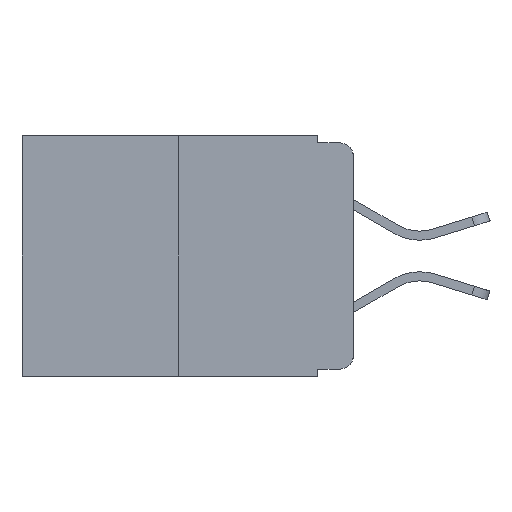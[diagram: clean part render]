
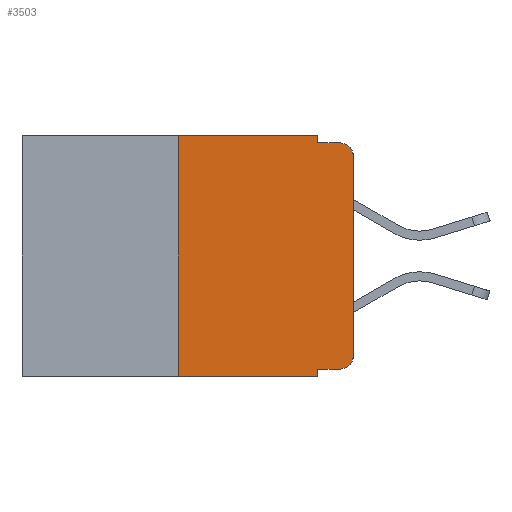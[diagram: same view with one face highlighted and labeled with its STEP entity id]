
A CAD part, left-side view. The second image highlights one B-rep face of the part: STEP entity #3503.
In plain terms, the highlighted planar face has unit normal (-1, 0, 0).
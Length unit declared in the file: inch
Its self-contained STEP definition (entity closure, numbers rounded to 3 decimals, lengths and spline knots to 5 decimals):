
#55 = LINE ( 'NONE', #13478, #4183 ) ;
#272 = DIRECTION ( 'NONE',  ( 0., 0., 1. ) ) ;
#337 = AXIS2_PLACEMENT_3D ( 'NONE', #536, #3952, #6984 ) ;
#490 = ORIENTED_EDGE ( 'NONE', *, *, #3819, .T. ) ;
#536 = CARTESIAN_POINT ( 'NONE',  ( 0., 0.02, -0.313 ) ) ;
#704 = DIRECTION ( 'NONE',  ( 1., 0., 0. ) ) ;
#1139 = AXIS2_PLACEMENT_3D ( 'NONE', #10734, #704, #8183 ) ;
#1156 = VERTEX_POINT ( 'NONE', #13085 ) ;
#1263 = CARTESIAN_POINT ( 'NONE',  ( 0., 0.051, -0.01 ) ) ;
#1621 = CARTESIAN_POINT ( 'NONE',  ( 0., 0., -0.03 ) ) ;
#1637 = CARTESIAN_POINT ( 'NONE',  ( 0., 0.25, -0.343 ) ) ;
#1801 = PLANE ( 'NONE',  #1139 ) ;
#2365 = DIRECTION ( 'NONE',  ( 0., -1., 0. ) ) ;
#2472 = DIRECTION ( 'NONE',  ( 0., -1., 0. ) ) ;
#2976 = VERTEX_POINT ( 'NONE', #6078 ) ;
#3007 = DIRECTION ( 'NONE',  ( 0., 0., -1. ) ) ;
#3343 = VERTEX_POINT ( 'NONE', #11411 ) ;
#3503 = ADVANCED_FACE ( 'NONE', ( #11851 ), #1801, .F. ) ;
#3701 = ORIENTED_EDGE ( 'NONE', *, *, #7362, .T. ) ;
#3819 = EDGE_CURVE ( 'NONE', #2976, #9929, #55, .T. ) ;
#3894 = CARTESIAN_POINT ( 'NONE',  ( 0., 0.02, -0.333 ) ) ;
#3932 = VERTEX_POINT ( 'NONE', #1637 ) ;
#3952 = DIRECTION ( 'NONE',  ( -1., 0., 0. ) ) ;
#4183 = VECTOR ( 'NONE', #272, 39.37008 ) ;
#4614 = AXIS2_PLACEMENT_3D ( 'NONE', #6065, #12837, #7255 ) ;
#4623 = LINE ( 'NONE', #1263, #12595 ) ;
#4680 = ORIENTED_EDGE ( 'NONE', *, *, #5674, .F. ) ;
#5674 = EDGE_CURVE ( 'NONE', #7776, #1156, #10786, .T. ) ;
#6061 = CARTESIAN_POINT ( 'NONE',  ( 0., 0.051, 0. ) ) ;
#6065 = CARTESIAN_POINT ( 'NONE',  ( 0., 0.02, -0.03 ) ) ;
#6078 = CARTESIAN_POINT ( 'NONE',  ( 0., 0., -0.313 ) ) ;
#6122 = CARTESIAN_POINT ( 'NONE',  ( 0., 0.473, -0.343 ) ) ;
#6129 = EDGE_CURVE ( 'NONE', #6650, #11238, #13418, .T. ) ;
#6491 = CIRCLE ( 'NONE', #4614, 0.02 ) ;
#6640 = VECTOR ( 'NONE', #7541, 39.37008 ) ;
#6650 = VERTEX_POINT ( 'NONE', #7883 ) ;
#6685 = ORIENTED_EDGE ( 'NONE', *, *, #8653, .F. ) ;
#6984 = DIRECTION ( 'NONE',  ( 0., 0., -1. ) ) ;
#7255 = DIRECTION ( 'NONE',  ( 0., 0., -1. ) ) ;
#7257 = ORIENTED_EDGE ( 'NONE', *, *, #11664, .T. ) ;
#7299 = VERTEX_POINT ( 'NONE', #10491 ) ;
#7362 = EDGE_CURVE ( 'NONE', #11238, #2976, #8050, .T. ) ;
#7425 = EDGE_CURVE ( 'NONE', #11538, #7776, #13063, .T. ) ;
#7454 = CARTESIAN_POINT ( 'NONE',  ( 0., 0.25, 0. ) ) ;
#7541 = DIRECTION ( 'NONE',  ( 0., -1., 0. ) ) ;
#7776 = VERTEX_POINT ( 'NONE', #6061 ) ;
#7883 = CARTESIAN_POINT ( 'NONE',  ( 0., 0.051, -0.333 ) ) ;
#8050 = CIRCLE ( 'NONE', #337, 0.02 ) ;
#8183 = DIRECTION ( 'NONE',  ( 0., 0., -1. ) ) ;
#8188 = LINE ( 'NONE', #6122, #14429 ) ;
#8644 = DIRECTION ( 'NONE',  ( 0., -1., 0. ) ) ;
#8653 = EDGE_CURVE ( 'NONE', #6650, #7299, #9460, .T. ) ;
#9460 = LINE ( 'NONE', #11605, #11350 ) ;
#9487 = EDGE_CURVE ( 'NONE', #3932, #7299, #8188, .T. ) ;
#9598 = CARTESIAN_POINT ( 'NONE',  ( 0., 0.473, 0. ) ) ;
#9722 = EDGE_LOOP ( 'NONE', ( #490, #7257, #13806, #4680, #13433, #13866, #10320, #6685, #13300, #3701 ) ) ;
#9912 = CARTESIAN_POINT ( 'NONE',  ( 0., 0.051, 0. ) ) ;
#9929 = VERTEX_POINT ( 'NONE', #1621 ) ;
#10320 = ORIENTED_EDGE ( 'NONE', *, *, #9487, .T. ) ;
#10491 = CARTESIAN_POINT ( 'NONE',  ( 0., 0.051, -0.343 ) ) ;
#10734 = CARTESIAN_POINT ( 'NONE',  ( 0., 0.473, 0. ) ) ;
#10786 = LINE ( 'NONE', #9912, #13117 ) ;
#10960 = EDGE_CURVE ( 'NONE', #1156, #3343, #4623, .T. ) ;
#11035 = CARTESIAN_POINT ( 'NONE',  ( 0., 0.051, -0.333 ) ) ;
#11238 = VERTEX_POINT ( 'NONE', #3894 ) ;
#11252 = VECTOR ( 'NONE', #11927, 39.37008 ) ;
#11326 = VECTOR ( 'NONE', #8644, 39.37008 ) ;
#11350 = VECTOR ( 'NONE', #14027, 39.37008 ) ;
#11411 = CARTESIAN_POINT ( 'NONE',  ( 0., 0.02, -0.01 ) ) ;
#11538 = VERTEX_POINT ( 'NONE', #12254 ) ;
#11605 = CARTESIAN_POINT ( 'NONE',  ( 0., 0.051, 0. ) ) ;
#11664 = EDGE_CURVE ( 'NONE', #9929, #3343, #6491, .T. ) ;
#11851 = FACE_OUTER_BOUND ( 'NONE', #9722, .T. ) ;
#11927 = DIRECTION ( 'NONE',  ( 0., 0., 1. ) ) ;
#12254 = CARTESIAN_POINT ( 'NONE',  ( 0., 0.25, 0. ) ) ;
#12595 = VECTOR ( 'NONE', #2365, 39.37008 ) ;
#12837 = DIRECTION ( 'NONE',  ( -1., 0., 0. ) ) ;
#13063 = LINE ( 'NONE', #9598, #11326 ) ;
#13085 = CARTESIAN_POINT ( 'NONE',  ( 0., 0.051, -0.01 ) ) ;
#13117 = VECTOR ( 'NONE', #3007, 39.37008 ) ;
#13300 = ORIENTED_EDGE ( 'NONE', *, *, #6129, .T. ) ;
#13376 = EDGE_CURVE ( 'NONE', #3932, #11538, #14003, .T. ) ;
#13418 = LINE ( 'NONE', #11035, #6640 ) ;
#13433 = ORIENTED_EDGE ( 'NONE', *, *, #7425, .F. ) ;
#13478 = CARTESIAN_POINT ( 'NONE',  ( 0., 0., 0. ) ) ;
#13806 = ORIENTED_EDGE ( 'NONE', *, *, #10960, .F. ) ;
#13866 = ORIENTED_EDGE ( 'NONE', *, *, #13376, .F. ) ;
#14003 = LINE ( 'NONE', #7454, #11252 ) ;
#14027 = DIRECTION ( 'NONE',  ( 0., 0., -1. ) ) ;
#14429 = VECTOR ( 'NONE', #2472, 39.37008 ) ;
